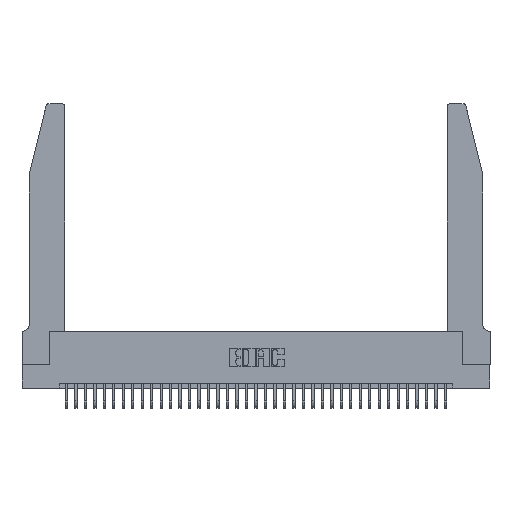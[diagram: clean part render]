
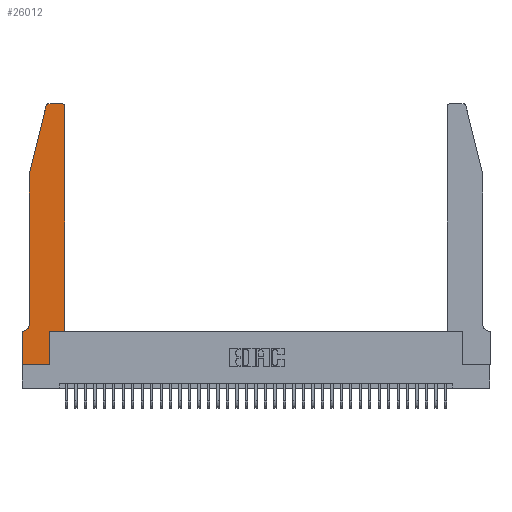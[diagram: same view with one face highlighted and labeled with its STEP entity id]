
A CAD part, top view. The second image highlights one B-rep face of the part: STEP entity #26012.
In plain terms, the highlighted planar face has unit normal (0, 0, 1).
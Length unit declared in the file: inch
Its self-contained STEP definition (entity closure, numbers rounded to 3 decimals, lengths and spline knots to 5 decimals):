
#120 = DIRECTION ( 'NONE',  ( 1., 0., 0. ) ) ;
#1638 = VERTEX_POINT ( 'NONE', #35002 ) ;
#1963 = ORIENTED_EDGE ( 'NONE', *, *, #16748, .T. ) ;
#2654 = DIRECTION ( 'NONE',  ( -1., 0., 0. ) ) ;
#3295 = CARTESIAN_POINT ( 'NONE',  ( 0., 0.35, 0.37 ) ) ;
#3702 = CARTESIAN_POINT ( 'NONE',  ( 0.4505, 0.35, 0.37 ) ) ;
#3862 = LINE ( 'NONE', #14707, #25931 ) ;
#4063 = CIRCLE ( 'NONE', #37566, 0.07 ) ;
#4165 = CARTESIAN_POINT ( 'NONE',  ( 0., 0., 0.37 ) ) ;
#4360 = DIRECTION ( 'NONE',  ( 0., 1., 0. ) ) ;
#5798 = DIRECTION ( 'NONE',  ( -1., 0., 0. ) ) ;
#6271 = VECTOR ( 'NONE', #24339, 39.37008 ) ;
#6287 = DIRECTION ( 'NONE',  ( 1., 0., 0. ) ) ;
#6441 = CARTESIAN_POINT ( 'NONE',  ( 0.0755, 2., 0.37 ) ) ;
#6645 = ORIENTED_EDGE ( 'NONE', *, *, #22093, .T. ) ;
#6734 = DIRECTION ( 'NONE',  ( -1., 0., 0. ) ) ;
#7146 = VERTEX_POINT ( 'NONE', #11273 ) ;
#7606 = ORIENTED_EDGE ( 'NONE', *, *, #26971, .T. ) ;
#8354 = DIRECTION ( 'NONE',  ( 1., 0., 0. ) ) ;
#8736 = LINE ( 'NONE', #33744, #17689 ) ;
#9007 = ORIENTED_EDGE ( 'NONE', *, *, #17328, .T. ) ;
#9480 = ORIENTED_EDGE ( 'NONE', *, *, #36322, .T. ) ;
#9684 = CARTESIAN_POINT ( 'NONE',  ( 0.25487, 2.72718, 0.37 ) ) ;
#9938 = LINE ( 'NONE', #23807, #26861 ) ;
#10007 = VERTEX_POINT ( 'NONE', #10213 ) ;
#10213 = CARTESIAN_POINT ( 'NONE',  ( 0., 0.35, 0.37 ) ) ;
#10519 = AXIS2_PLACEMENT_3D ( 'NONE', #10841, #31811, #13886 ) ;
#10841 = CARTESIAN_POINT ( 'NONE',  ( 0.4205, 2.72, 0.37 ) ) ;
#11273 = CARTESIAN_POINT ( 'NONE',  ( 0.0755, 0.42, 0.37 ) ) ;
#11806 = VERTEX_POINT ( 'NONE', #9684 ) ;
#11849 = ORIENTED_EDGE ( 'NONE', *, *, #33126, .T. ) ;
#12081 = VERTEX_POINT ( 'NONE', #30529 ) ;
#12106 = CARTESIAN_POINT ( 'NONE',  ( 0.284, 2.75, 0.37 ) ) ;
#12238 = VERTEX_POINT ( 'NONE', #13494 ) ;
#12319 = CARTESIAN_POINT ( 'NONE',  ( 0.4505, 0.35, 0.37 ) ) ;
#12337 = ORIENTED_EDGE ( 'NONE', *, *, #14207, .T. ) ;
#12565 = CIRCLE ( 'NONE', #17386, 0.03 ) ;
#12785 = ORIENTED_EDGE ( 'NONE', *, *, #30280, .T. ) ;
#12856 = VECTOR ( 'NONE', #4360, 39.37008 ) ;
#13494 = CARTESIAN_POINT ( 'NONE',  ( 0.4205, 2.75, 0.37 ) ) ;
#13886 = DIRECTION ( 'NONE',  ( 1., 0., 0. ) ) ;
#14207 = EDGE_CURVE ( 'NONE', #1638, #12238, #20694, .T. ) ;
#14679 = ORIENTED_EDGE ( 'NONE', *, *, #31141, .T. ) ;
#14707 = CARTESIAN_POINT ( 'NONE',  ( 0.2865, 0.35, 0.37 ) ) ;
#14838 = VECTOR ( 'NONE', #34051, 39.37008 ) ;
#14857 = CARTESIAN_POINT ( 'NONE',  ( 0.0755, 2., 0.37 ) ) ;
#15765 = VECTOR ( 'NONE', #8354, 39.37008 ) ;
#16350 = CARTESIAN_POINT ( 'NONE',  ( 0.4505, 0.35, 0.37 ) ) ;
#16748 = EDGE_CURVE ( 'NONE', #28358, #11806, #12565, .T. ) ;
#17328 = EDGE_CURVE ( 'NONE', #12238, #28358, #8736, .T. ) ;
#17386 = AXIS2_PLACEMENT_3D ( 'NONE', #35967, #18125, #120 ) ;
#17689 = VECTOR ( 'NONE', #6734, 39.37008 ) ;
#18125 = DIRECTION ( 'NONE',  ( 0., 0., 1. ) ) ;
#18547 = EDGE_CURVE ( 'NONE', #11806, #30862, #30247, .T. ) ;
#18827 = EDGE_CURVE ( 'NONE', #27956, #1638, #28822, .T. ) ;
#20468 = LINE ( 'NONE', #12319, #29376 ) ;
#20666 = DIRECTION ( 'NONE',  ( 0., 0., -1. ) ) ;
#20694 = CIRCLE ( 'NONE', #10519, 0.03 ) ;
#21352 = CARTESIAN_POINT ( 'NONE',  ( 0.0755, 2., 0.37 ) ) ;
#21394 = DIRECTION ( 'NONE',  ( 1., 0., 0. ) ) ;
#22093 = EDGE_CURVE ( 'NONE', #26396, #10007, #9938, .T. ) ;
#22820 = LINE ( 'NONE', #4165, #14838 ) ;
#23744 = DIRECTION ( 'NONE',  ( 0., 1., 0. ) ) ;
#23759 = VERTEX_POINT ( 'NONE', #25604 ) ;
#23807 = CARTESIAN_POINT ( 'NONE',  ( 0.0755, 0.35, 0.37 ) ) ;
#24196 = FACE_OUTER_BOUND ( 'NONE', #35218, .T. ) ;
#24292 = DIRECTION ( 'NONE',  ( 0., 0., 1. ) ) ;
#24339 = DIRECTION ( 'NONE',  ( -0.239, -0.971, 0. ) ) ;
#25604 = CARTESIAN_POINT ( 'NONE',  ( 0.2865, 0.35, 0.37 ) ) ;
#25903 = ORIENTED_EDGE ( 'NONE', *, *, #18547, .T. ) ;
#25931 = VECTOR ( 'NONE', #23744, 39.37008 ) ;
#26012 = ADVANCED_FACE ( 'NONE', ( #24196 ), #30198, .T. ) ;
#26396 = VERTEX_POINT ( 'NONE', #28990 ) ;
#26861 = VECTOR ( 'NONE', #5798, 39.37008 ) ;
#26971 = EDGE_CURVE ( 'NONE', #30153, #12081, #31663, .T. ) ;
#27348 = ORIENTED_EDGE ( 'NONE', *, *, #18827, .T. ) ;
#27956 = VERTEX_POINT ( 'NONE', #3702 ) ;
#28358 = VERTEX_POINT ( 'NONE', #12106 ) ;
#28822 = LINE ( 'NONE', #16350, #12856 ) ;
#28920 = CARTESIAN_POINT ( 'NONE',  ( 0., 0., 0.37 ) ) ;
#28990 = CARTESIAN_POINT ( 'NONE',  ( 0.0055, 0.35, 0.37 ) ) ;
#29234 = CARTESIAN_POINT ( 'NONE',  ( 0., 0., 0.37 ) ) ;
#29376 = VECTOR ( 'NONE', #21394, 39.37008 ) ;
#29379 = AXIS2_PLACEMENT_3D ( 'NONE', #3295, #24292, #6287 ) ;
#30153 = VERTEX_POINT ( 'NONE', #28920 ) ;
#30198 = PLANE ( 'NONE',  #29379 ) ;
#30247 = LINE ( 'NONE', #21352, #6271 ) ;
#30280 = EDGE_CURVE ( 'NONE', #7146, #26396, #4063, .T. ) ;
#30529 = CARTESIAN_POINT ( 'NONE',  ( 0.2865, 0., 0.37 ) ) ;
#30862 = VERTEX_POINT ( 'NONE', #14857 ) ;
#31141 = EDGE_CURVE ( 'NONE', #10007, #30153, #22820, .T. ) ;
#31663 = LINE ( 'NONE', #29234, #15765 ) ;
#31811 = DIRECTION ( 'NONE',  ( 0., 0., 1. ) ) ;
#32462 = ORIENTED_EDGE ( 'NONE', *, *, #38009, .T. ) ;
#32514 = VECTOR ( 'NONE', #36404, 39.37008 ) ;
#33126 = EDGE_CURVE ( 'NONE', #30862, #7146, #33459, .T. ) ;
#33459 = LINE ( 'NONE', #6441, #32514 ) ;
#33744 = CARTESIAN_POINT ( 'NONE',  ( 0.2605, 2.75, 0.37 ) ) ;
#34051 = DIRECTION ( 'NONE',  ( 0., -1., 0. ) ) ;
#35002 = CARTESIAN_POINT ( 'NONE',  ( 0.4505, 2.72, 0.37 ) ) ;
#35218 = EDGE_LOOP ( 'NONE', ( #9007, #1963, #25903, #11849, #12785, #6645, #14679, #7606, #32462, #9480, #27348, #12337 ) ) ;
#35967 = CARTESIAN_POINT ( 'NONE',  ( 0.284, 2.72, 0.37 ) ) ;
#36322 = EDGE_CURVE ( 'NONE', #23759, #27956, #20468, .T. ) ;
#36404 = DIRECTION ( 'NONE',  ( 0., -1., 0. ) ) ;
#37566 = AXIS2_PLACEMENT_3D ( 'NONE', #38484, #20666, #2654 ) ;
#38009 = EDGE_CURVE ( 'NONE', #12081, #23759, #3862, .T. ) ;
#38484 = CARTESIAN_POINT ( 'NONE',  ( 0.0055, 0.42, 0.37 ) ) ;
